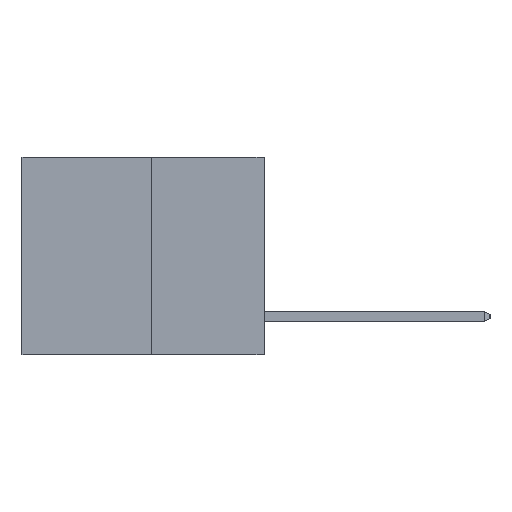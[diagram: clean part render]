
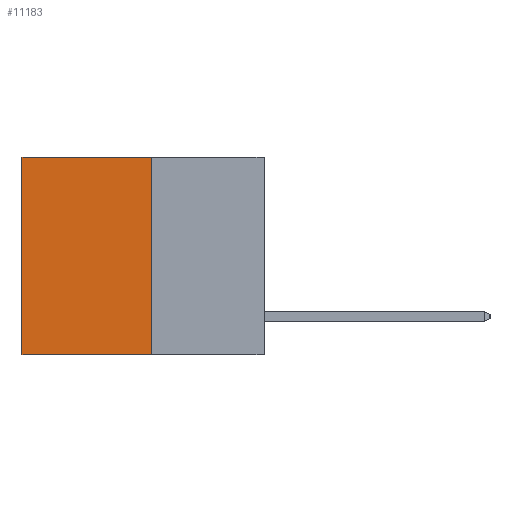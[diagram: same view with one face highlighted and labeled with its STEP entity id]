
A CAD part, left-side view. The second image highlights one B-rep face of the part: STEP entity #11183.
In plain terms, the highlighted planar face has unit normal (-1, 0, 0).
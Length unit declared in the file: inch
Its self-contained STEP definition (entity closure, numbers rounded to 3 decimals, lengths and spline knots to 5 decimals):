
#417 = FACE_OUTER_BOUND ( 'NONE', #16708, .T. ) ;
#718 = LINE ( 'NONE', #3241, #15012 ) ;
#722 = VERTEX_POINT ( 'NONE', #15738 ) ;
#845 = EDGE_CURVE ( 'NONE', #722, #15480, #718, .T. ) ;
#1965 = ORIENTED_EDGE ( 'NONE', *, *, #7141, .T. ) ;
#2000 = ORIENTED_EDGE ( 'NONE', *, *, #845, .F. ) ;
#2069 = LINE ( 'NONE', #15169, #5183 ) ;
#2383 = PLANE ( 'NONE',  #3866 ) ;
#3241 = CARTESIAN_POINT ( 'NONE',  ( 0.3165, 0.28, -0.49 ) ) ;
#3866 = AXIS2_PLACEMENT_3D ( 'NONE', #16416, #12321, #7821 ) ;
#4263 = DIRECTION ( 'NONE',  ( 0., 1., 0. ) ) ;
#4356 = VERTEX_POINT ( 'NONE', #6697 ) ;
#5183 = VECTOR ( 'NONE', #6831, 39.37008 ) ;
#6661 = LINE ( 'NONE', #10171, #6868 ) ;
#6697 = CARTESIAN_POINT ( 'NONE',  ( 0.3165, 0.28, 0. ) ) ;
#6831 = DIRECTION ( 'NONE',  ( 0., 0., -1. ) ) ;
#6868 = VECTOR ( 'NONE', #13039, 39.37008 ) ;
#7141 = EDGE_CURVE ( 'NONE', #4356, #12403, #14263, .T. ) ;
#7526 = VECTOR ( 'NONE', #4263, 39.37008 ) ;
#7821 = DIRECTION ( 'NONE',  ( 0., 0., -1. ) ) ;
#8489 = CARTESIAN_POINT ( 'NONE',  ( 0.3165, 0.6, 0. ) ) ;
#9374 = CARTESIAN_POINT ( 'NONE',  ( 0.3165, 0.6, -0.49 ) ) ;
#10171 = CARTESIAN_POINT ( 'NONE',  ( 0.3165, 0.6, -0.49 ) ) ;
#10856 = EDGE_CURVE ( 'NONE', #12403, #15480, #6661, .T. ) ;
#11183 = ADVANCED_FACE ( 'NONE', ( #417 ), #2383, .F. ) ;
#12159 = ORIENTED_EDGE ( 'NONE', *, *, #15679, .F. ) ;
#12321 = DIRECTION ( 'NONE',  ( 1., 0., 0. ) ) ;
#12403 = VERTEX_POINT ( 'NONE', #8489 ) ;
#13039 = DIRECTION ( 'NONE',  ( 0., 0., -1. ) ) ;
#14263 = LINE ( 'NONE', #18315, #7526 ) ;
#15012 = VECTOR ( 'NONE', #17541, 39.37008 ) ;
#15169 = CARTESIAN_POINT ( 'NONE',  ( 0.3165, 0.28, -0.49 ) ) ;
#15480 = VERTEX_POINT ( 'NONE', #9374 ) ;
#15679 = EDGE_CURVE ( 'NONE', #4356, #722, #2069, .T. ) ;
#15738 = CARTESIAN_POINT ( 'NONE',  ( 0.3165, 0.28, -0.49 ) ) ;
#16416 = CARTESIAN_POINT ( 'NONE',  ( 0.3165, 0.28, -0.49 ) ) ;
#16708 = EDGE_LOOP ( 'NONE', ( #17312, #2000, #12159, #1965 ) ) ;
#17312 = ORIENTED_EDGE ( 'NONE', *, *, #10856, .T. ) ;
#17541 = DIRECTION ( 'NONE',  ( 0., 1., 0. ) ) ;
#18315 = CARTESIAN_POINT ( 'NONE',  ( 0.3165, 0.28, 0. ) ) ;
